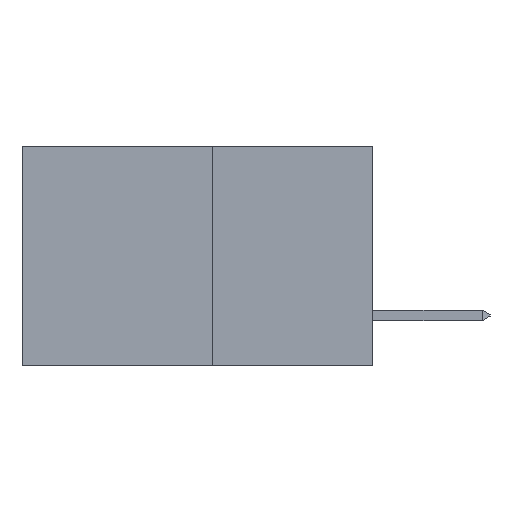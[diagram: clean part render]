
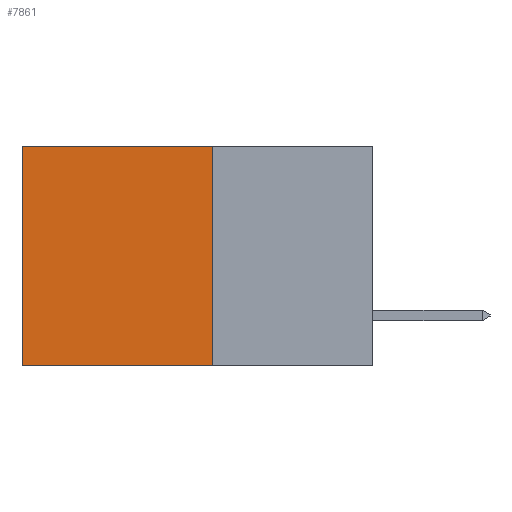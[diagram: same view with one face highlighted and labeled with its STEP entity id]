
A CAD part, left-side view. The second image highlights one B-rep face of the part: STEP entity #7861.
In plain terms, the highlighted planar face has unit normal (-1, 0, 0).
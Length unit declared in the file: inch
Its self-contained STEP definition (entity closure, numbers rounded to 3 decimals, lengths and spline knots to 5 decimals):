
#107 = VERTEX_POINT ( 'NONE', #2951 ) ;
#368 = VERTEX_POINT ( 'NONE', #9400 ) ;
#673 = AXIS2_PLACEMENT_3D ( 'NONE', #11004, #8403, #2855 ) ;
#881 = LINE ( 'NONE', #1767, #5242 ) ;
#886 = EDGE_CURVE ( 'NONE', #368, #107, #9741, .T. ) ;
#1767 = CARTESIAN_POINT ( 'NONE',  ( 0.277, 0.27, 0. ) ) ;
#1933 = PLANE ( 'NONE',  #673 ) ;
#2073 = DIRECTION ( 'NONE',  ( 0., 1., 0. ) ) ;
#2169 = EDGE_LOOP ( 'NONE', ( #4191, #10915, #10154, #11317 ) ) ;
#2349 = LINE ( 'NONE', #5716, #9137 ) ;
#2415 = VECTOR ( 'NONE', #4453, 39.37008 ) ;
#2534 = CARTESIAN_POINT ( 'NONE',  ( 0.277, 0.59, 0. ) ) ;
#2855 = DIRECTION ( 'NONE',  ( 0., 0., -1. ) ) ;
#2904 = CARTESIAN_POINT ( 'NONE',  ( 0.277, 0.27, -0.37 ) ) ;
#2951 = CARTESIAN_POINT ( 'NONE',  ( 0.277, 0.27, -0.37 ) ) ;
#3022 = VECTOR ( 'NONE', #2073, 39.37008 ) ;
#3583 = EDGE_CURVE ( 'NONE', #6020, #8938, #2349, .T. ) ;
#4191 = ORIENTED_EDGE ( 'NONE', *, *, #3583, .T. ) ;
#4453 = DIRECTION ( 'NONE',  ( 0., 0., -1. ) ) ;
#5242 = VECTOR ( 'NONE', #6382, 39.37008 ) ;
#5430 = EDGE_CURVE ( 'NONE', #107, #8938, #5496, .T. ) ;
#5496 = LINE ( 'NONE', #2904, #3022 ) ;
#5716 = CARTESIAN_POINT ( 'NONE',  ( 0.277, 0.59, -0.37 ) ) ;
#5976 = DIRECTION ( 'NONE',  ( 0., 0., -1. ) ) ;
#6020 = VERTEX_POINT ( 'NONE', #2534 ) ;
#6382 = DIRECTION ( 'NONE',  ( 0., 1., 0. ) ) ;
#7768 = CARTESIAN_POINT ( 'NONE',  ( 0.277, 0.27, -0.37 ) ) ;
#7861 = ADVANCED_FACE ( 'NONE', ( #11489 ), #1933, .F. ) ;
#8403 = DIRECTION ( 'NONE',  ( 1., 0., 0. ) ) ;
#8938 = VERTEX_POINT ( 'NONE', #9863 ) ;
#9137 = VECTOR ( 'NONE', #5976, 39.37008 ) ;
#9400 = CARTESIAN_POINT ( 'NONE',  ( 0.277, 0.27, 0. ) ) ;
#9741 = LINE ( 'NONE', #7768, #2415 ) ;
#9863 = CARTESIAN_POINT ( 'NONE',  ( 0.277, 0.59, -0.37 ) ) ;
#10154 = ORIENTED_EDGE ( 'NONE', *, *, #886, .F. ) ;
#10762 = EDGE_CURVE ( 'NONE', #368, #6020, #881, .T. ) ;
#10915 = ORIENTED_EDGE ( 'NONE', *, *, #5430, .F. ) ;
#11004 = CARTESIAN_POINT ( 'NONE',  ( 0.277, 0.27, -0.37 ) ) ;
#11317 = ORIENTED_EDGE ( 'NONE', *, *, #10762, .T. ) ;
#11489 = FACE_OUTER_BOUND ( 'NONE', #2169, .T. ) ;
